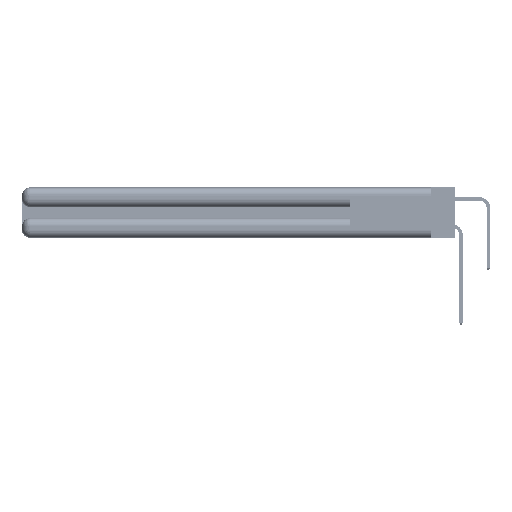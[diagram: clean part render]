
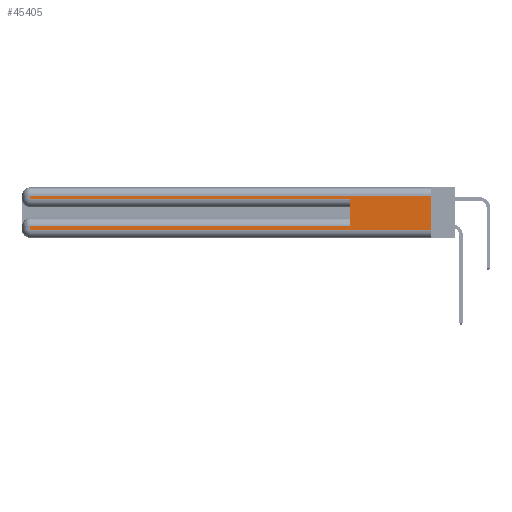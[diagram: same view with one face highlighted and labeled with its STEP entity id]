
A CAD part, left-side view. The second image highlights one B-rep face of the part: STEP entity #45405.
In plain terms, the highlighted planar face has unit normal (-1, 0, 0).
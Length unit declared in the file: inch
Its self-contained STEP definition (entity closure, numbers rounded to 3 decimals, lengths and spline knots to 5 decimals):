
#95 = CARTESIAN_POINT ( 'NONE',  ( 0., 0., 0.06 ) ) ;
#1691 = VERTEX_POINT ( 'NONE', #30272 ) ;
#1947 = DIRECTION ( 'NONE',  ( 0., 1., 0. ) ) ;
#2159 = VERTEX_POINT ( 'NONE', #15676 ) ;
#2589 = VECTOR ( 'NONE', #5786, 39.37008 ) ;
#3121 = ORIENTED_EDGE ( 'NONE', *, *, #43541, .T. ) ;
#3735 = CARTESIAN_POINT ( 'NONE',  ( 0., 2.94, 0.06 ) ) ;
#5786 = DIRECTION ( 'NONE',  ( 0., 0., -1. ) ) ;
#6182 = EDGE_CURVE ( 'NONE', #16410, #38180, #57744, .T. ) ;
#6590 = CARTESIAN_POINT ( 'NONE',  ( 0., 2.94, 0.37 ) ) ;
#6948 = CARTESIAN_POINT ( 'NONE',  ( 0., 0., 0.31 ) ) ;
#7766 = EDGE_CURVE ( 'NONE', #32370, #24507, #48578, .T. ) ;
#8971 = VECTOR ( 'NONE', #19551, 39.37008 ) ;
#9998 = EDGE_CURVE ( 'NONE', #24507, #16410, #31500, .T. ) ;
#10354 = CARTESIAN_POINT ( 'NONE',  ( 0., 0., 0.37 ) ) ;
#13799 = CARTESIAN_POINT ( 'NONE',  ( 0., 0., 0.285 ) ) ;
#15676 = CARTESIAN_POINT ( 'NONE',  ( 0., 0.6, 0.285 ) ) ;
#16410 = VERTEX_POINT ( 'NONE', #3735 ) ;
#19209 = CARTESIAN_POINT ( 'NONE',  ( 0., 0., 0.37 ) ) ;
#19349 = ORIENTED_EDGE ( 'NONE', *, *, #53647, .T. ) ;
#19551 = DIRECTION ( 'NONE',  ( 0., 0., -1. ) ) ;
#21457 = ORIENTED_EDGE ( 'NONE', *, *, #33452, .T. ) ;
#22016 = VECTOR ( 'NONE', #36137, 39.37008 ) ;
#22482 = CARTESIAN_POINT ( 'NONE',  ( 0., 0., 0.06 ) ) ;
#23324 = CARTESIAN_POINT ( 'NONE',  ( 0., 0.6, 0.145 ) ) ;
#23955 = DIRECTION ( 'NONE',  ( 1., 0., 0. ) ) ;
#24507 = VERTEX_POINT ( 'NONE', #48259 ) ;
#26041 = FACE_OUTER_BOUND ( 'NONE', #37840, .T. ) ;
#27391 = VECTOR ( 'NONE', #27846, 39.37008 ) ;
#27846 = DIRECTION ( 'NONE',  ( 0., 0., 1. ) ) ;
#29077 = VECTOR ( 'NONE', #38083, 39.37008 ) ;
#29224 = ORIENTED_EDGE ( 'NONE', *, *, #35668, .F. ) ;
#30272 = CARTESIAN_POINT ( 'NONE',  ( 0., 2.94, 0.285 ) ) ;
#30676 = ORIENTED_EDGE ( 'NONE', *, *, #6182, .T. ) ;
#31500 = LINE ( 'NONE', #46388, #8971 ) ;
#32370 = VERTEX_POINT ( 'NONE', #34031 ) ;
#33444 = CARTESIAN_POINT ( 'NONE',  ( 0., 0., 0.085 ) ) ;
#33452 = EDGE_CURVE ( 'NONE', #55520, #48410, #35407, .T. ) ;
#34031 = CARTESIAN_POINT ( 'NONE',  ( 0., 0.6, 0.085 ) ) ;
#35407 = LINE ( 'NONE', #6948, #47295 ) ;
#35480 = ORIENTED_EDGE ( 'NONE', *, *, #57417, .F. ) ;
#35668 = EDGE_CURVE ( 'NONE', #32370, #2159, #37942, .T. ) ;
#36137 = DIRECTION ( 'NONE',  ( 0., -1., 0. ) ) ;
#36258 = VECTOR ( 'NONE', #45210, 39.37008 ) ;
#36672 = VECTOR ( 'NONE', #1947, 39.37008 ) ;
#37311 = PLANE ( 'NONE',  #51680 ) ;
#37840 = EDGE_LOOP ( 'NONE', ( #35480, #21457, #3121, #19349, #29224, #46727, #40426, #30676 ) ) ;
#37873 = CARTESIAN_POINT ( 'NONE',  ( 0., 0., 0.31 ) ) ;
#37942 = LINE ( 'NONE', #23324, #27391 ) ;
#38083 = DIRECTION ( 'NONE',  ( 0., 0., -1. ) ) ;
#38180 = VERTEX_POINT ( 'NONE', #22482 ) ;
#38419 = DIRECTION ( 'NONE',  ( 0., 1., 0. ) ) ;
#39587 = LINE ( 'NONE', #6590, #29077 ) ;
#40426 = ORIENTED_EDGE ( 'NONE', *, *, #9998, .T. ) ;
#43318 = CARTESIAN_POINT ( 'NONE',  ( 0., 2.94, 0.31 ) ) ;
#43541 = EDGE_CURVE ( 'NONE', #48410, #1691, #39587, .T. ) ;
#45210 = DIRECTION ( 'NONE',  ( 0., -1., 0. ) ) ;
#45405 = ADVANCED_FACE ( 'NONE', ( #26041 ), #37311, .F. ) ;
#46388 = CARTESIAN_POINT ( 'NONE',  ( 0., 2.94, 0.37 ) ) ;
#46727 = ORIENTED_EDGE ( 'NONE', *, *, #7766, .T. ) ;
#46750 = LINE ( 'NONE', #13799, #36258 ) ;
#47295 = VECTOR ( 'NONE', #38419, 39.37008 ) ;
#48259 = CARTESIAN_POINT ( 'NONE',  ( 0., 2.94, 0.085 ) ) ;
#48410 = VERTEX_POINT ( 'NONE', #43318 ) ;
#48578 = LINE ( 'NONE', #33444, #36672 ) ;
#48959 = LINE ( 'NONE', #19209, #2589 ) ;
#51680 = AXIS2_PLACEMENT_3D ( 'NONE', #10354, #23955, #55268 ) ;
#53647 = EDGE_CURVE ( 'NONE', #1691, #2159, #46750, .T. ) ;
#55268 = DIRECTION ( 'NONE',  ( 0., 0., -1. ) ) ;
#55520 = VERTEX_POINT ( 'NONE', #37873 ) ;
#57417 = EDGE_CURVE ( 'NONE', #55520, #38180, #48959, .T. ) ;
#57744 = LINE ( 'NONE', #95, #22016 ) ;
